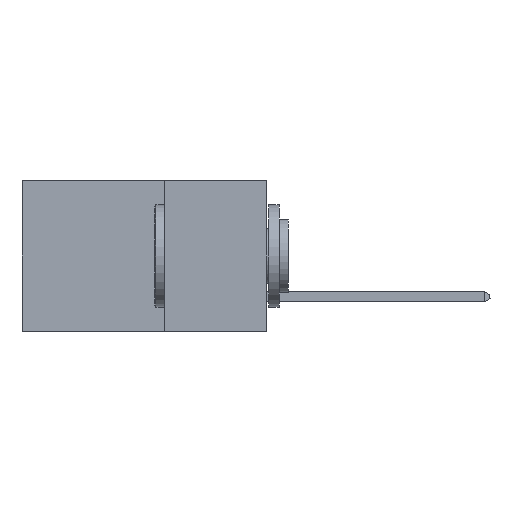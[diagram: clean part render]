
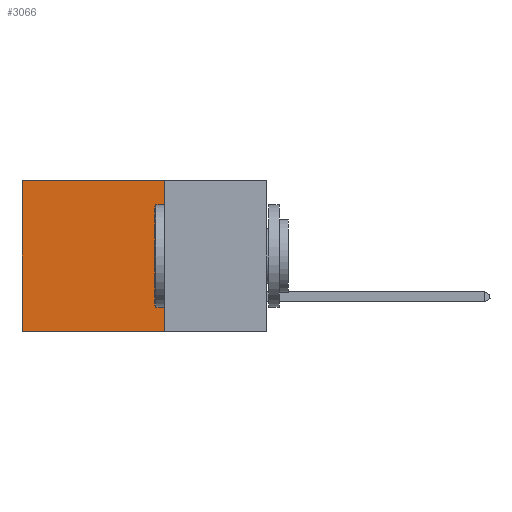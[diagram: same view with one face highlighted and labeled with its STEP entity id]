
A CAD part, left-side view. The second image highlights one B-rep face of the part: STEP entity #3066.
In plain terms, the highlighted planar face has unit normal (-1, 0, 0).
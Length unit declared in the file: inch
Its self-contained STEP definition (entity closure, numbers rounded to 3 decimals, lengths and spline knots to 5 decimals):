
#1365 = CARTESIAN_POINT ( 'NONE',  ( 0.2875, 0.25, -0.37 ) ) ;
#1459 = LINE ( 'NONE', #15995, #32045 ) ;
#3066 = ADVANCED_FACE ( 'NONE', ( #26732 ), #7939, .F. ) ;
#3360 = EDGE_LOOP ( 'NONE', ( #15034, #28759, #14898, #12013 ) ) ;
#4390 = VECTOR ( 'NONE', #30621, 39.37008 ) ;
#4434 = CARTESIAN_POINT ( 'NONE',  ( 0.2875, 0.25, -0.37 ) ) ;
#5175 = DIRECTION ( 'NONE',  ( 0., 0., -1. ) ) ;
#6927 = CARTESIAN_POINT ( 'NONE',  ( 0.2875, 0.25, 0. ) ) ;
#7595 = DIRECTION ( 'NONE',  ( 1., 0., 0. ) ) ;
#7939 = PLANE ( 'NONE',  #27225 ) ;
#9848 = DIRECTION ( 'NONE',  ( 0., 0., -1. ) ) ;
#9909 = DIRECTION ( 'NONE',  ( 0., 1., 0. ) ) ;
#10495 = CARTESIAN_POINT ( 'NONE',  ( 0.2875, 0.25, 0. ) ) ;
#10591 = EDGE_CURVE ( 'NONE', #30828, #31912, #1459, .T. ) ;
#10922 = CARTESIAN_POINT ( 'NONE',  ( 0.2875, 0.6, -0.37 ) ) ;
#11981 = CARTESIAN_POINT ( 'NONE',  ( 0.2875, 0.6, 0. ) ) ;
#12013 = ORIENTED_EDGE ( 'NONE', *, *, #10591, .T. ) ;
#13004 = CARTESIAN_POINT ( 'NONE',  ( 0.2875, 0.25, 0. ) ) ;
#14898 = ORIENTED_EDGE ( 'NONE', *, *, #27775, .F. ) ;
#15034 = ORIENTED_EDGE ( 'NONE', *, *, #24924, .T. ) ;
#15539 = VECTOR ( 'NONE', #9909, 39.37008 ) ;
#15995 = CARTESIAN_POINT ( 'NONE',  ( 0.2875, 0.25, 0. ) ) ;
#18044 = LINE ( 'NONE', #6927, #31049 ) ;
#18650 = LINE ( 'NONE', #11981, #4390 ) ;
#19313 = LINE ( 'NONE', #4434, #15539 ) ;
#19570 = VERTEX_POINT ( 'NONE', #1365 ) ;
#23574 = VERTEX_POINT ( 'NONE', #10922 ) ;
#24924 = EDGE_CURVE ( 'NONE', #31912, #23574, #18650, .T. ) ;
#26732 = FACE_OUTER_BOUND ( 'NONE', #3360, .T. ) ;
#27225 = AXIS2_PLACEMENT_3D ( 'NONE', #13004, #7595, #5175 ) ;
#27775 = EDGE_CURVE ( 'NONE', #30828, #19570, #18044, .T. ) ;
#28741 = CARTESIAN_POINT ( 'NONE',  ( 0.2875, 0.6, 0. ) ) ;
#28759 = ORIENTED_EDGE ( 'NONE', *, *, #32838, .F. ) ;
#29440 = DIRECTION ( 'NONE',  ( 0., 1., 0. ) ) ;
#30621 = DIRECTION ( 'NONE',  ( 0., 0., -1. ) ) ;
#30828 = VERTEX_POINT ( 'NONE', #10495 ) ;
#31049 = VECTOR ( 'NONE', #9848, 39.37008 ) ;
#31912 = VERTEX_POINT ( 'NONE', #28741 ) ;
#32045 = VECTOR ( 'NONE', #29440, 39.37008 ) ;
#32838 = EDGE_CURVE ( 'NONE', #19570, #23574, #19313, .T. ) ;
